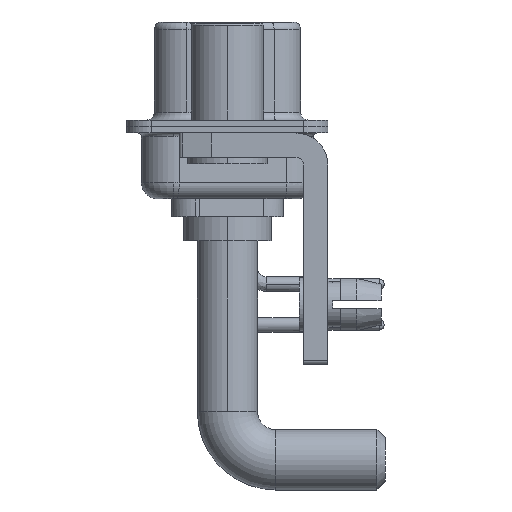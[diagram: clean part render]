
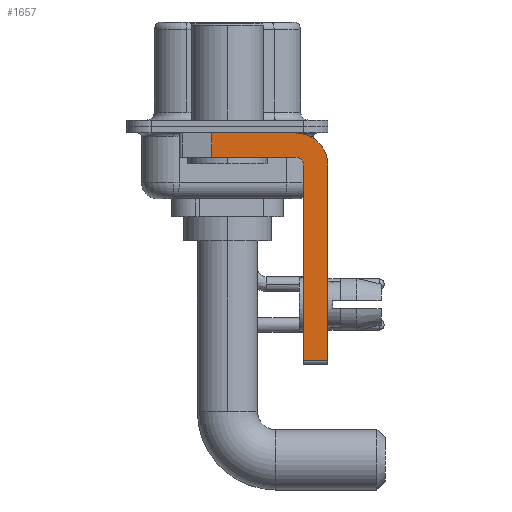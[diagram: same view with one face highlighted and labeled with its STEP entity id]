
A CAD part, left-side view. The second image highlights one B-rep face of the part: STEP entity #1657.
In plain terms, the highlighted planar face has unit normal (-1, 0, 0).
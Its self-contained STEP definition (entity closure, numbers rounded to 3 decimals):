
#322 = CARTESIAN_POINT ( 'NONE',  ( -2.9, -4.25, -1.9 ) ) ;
#999 = DIRECTION ( 'NONE',  ( 1., 0., 0. ) ) ;
#1108 = ORIENTED_EDGE ( 'NONE', *, *, #8049, .F. ) ;
#1657 = ADVANCED_FACE ( 'NONE', ( #18052 ), #25677, .F. ) ;
#1664 = CARTESIAN_POINT ( 'NONE',  ( -2.9, 0.978, -0.4 ) ) ;
#1812 = ORIENTED_EDGE ( 'NONE', *, *, #9223, .T. ) ;
#2180 = DIRECTION ( 'NONE',  ( 0., 0., -1. ) ) ;
#2213 = DIRECTION ( 'NONE',  ( 0., -1., 0. ) ) ;
#2520 = VERTEX_POINT ( 'NONE', #1664 ) ;
#2929 = CARTESIAN_POINT ( 'NONE',  ( -2.9, -4.25, -14.55 ) ) ;
#3032 = DIRECTION ( 'NONE',  ( 1., 0., 0. ) ) ;
#3142 = EDGE_LOOP ( 'NONE', ( #15228, #1812, #1108, #4092, #4650, #19514, #12246, #8804 ) ) ;
#3302 = CARTESIAN_POINT ( 'NONE',  ( -2.9, 0.978, -1.9 ) ) ;
#3963 = AXIS2_PLACEMENT_3D ( 'NONE', #21789, #3032, #10055 ) ;
#4092 = ORIENTED_EDGE ( 'NONE', *, *, #20405, .F. ) ;
#4118 = CARTESIAN_POINT ( 'NONE',  ( -2.9, -6.25, -14.55 ) ) ;
#4282 = CIRCLE ( 'NONE', #21753, 0.5 ) ;
#4650 = ORIENTED_EDGE ( 'NONE', *, *, #5585, .F. ) ;
#5585 = EDGE_CURVE ( 'NONE', #5754, #8852, #11050, .T. ) ;
#5587 = DIRECTION ( 'NONE',  ( 0., -1., 0. ) ) ;
#5754 = VERTEX_POINT ( 'NONE', #18016 ) ;
#6359 = DIRECTION ( 'NONE',  ( 0., 0., 1. ) ) ;
#8049 = EDGE_CURVE ( 'NONE', #29425, #20617, #15728, .T. ) ;
#8168 = DIRECTION ( 'NONE',  ( 0., 0., 1. ) ) ;
#8679 = CARTESIAN_POINT ( 'NONE',  ( -2.9, 0.978, -1.9 ) ) ;
#8804 = ORIENTED_EDGE ( 'NONE', *, *, #22685, .F. ) ;
#8818 = VECTOR ( 'NONE', #2213, 1000. ) ;
#8852 = VERTEX_POINT ( 'NONE', #23733 ) ;
#9223 = EDGE_CURVE ( 'NONE', #2520, #20617, #30101, .T. ) ;
#9384 = LINE ( 'NONE', #30484, #12333 ) ;
#9428 = AXIS2_PLACEMENT_3D ( 'NONE', #28188, #999, #27294 ) ;
#9888 = EDGE_CURVE ( 'NONE', #2520, #24561, #30674, .T. ) ;
#10055 = DIRECTION ( 'NONE',  ( 0., 0., -1. ) ) ;
#10423 = CARTESIAN_POINT ( 'NONE',  ( -2.9, -6.25, -2.4 ) ) ;
#11050 = LINE ( 'NONE', #20728, #16142 ) ;
#12246 = ORIENTED_EDGE ( 'NONE', *, *, #12914, .F. ) ;
#12333 = VECTOR ( 'NONE', #2180, 1000. ) ;
#12376 = CARTESIAN_POINT ( 'NONE',  ( -2.9, 3., -0.4 ) ) ;
#12457 = LINE ( 'NONE', #2929, #15855 ) ;
#12914 = EDGE_CURVE ( 'NONE', #25608, #18728, #9384, .T. ) ;
#13001 = CARTESIAN_POINT ( 'NONE',  ( -2.9, -4.25, -2.4 ) ) ;
#13775 = EDGE_CURVE ( 'NONE', #5754, #18728, #12457, .T. ) ;
#15228 = ORIENTED_EDGE ( 'NONE', *, *, #9888, .F. ) ;
#15265 = CARTESIAN_POINT ( 'NONE',  ( -2.9, -4.25, -1.9 ) ) ;
#15728 = LINE ( 'NONE', #15265, #21947 ) ;
#15855 = VECTOR ( 'NONE', #5587, 1000. ) ;
#16142 = VECTOR ( 'NONE', #6359, 1000. ) ;
#18016 = CARTESIAN_POINT ( 'NONE',  ( -2.9, -4.75, -14.55 ) ) ;
#18052 = FACE_OUTER_BOUND ( 'NONE', #3142, .T. ) ;
#18158 = CARTESIAN_POINT ( 'NONE',  ( -2.9, -4.25, -0.4 ) ) ;
#18465 = CIRCLE ( 'NONE', #3963, 2. ) ;
#18728 = VERTEX_POINT ( 'NONE', #4118 ) ;
#19514 = ORIENTED_EDGE ( 'NONE', *, *, #13775, .T. ) ;
#19955 = DIRECTION ( 'NONE',  ( 0., 0., -1. ) ) ;
#20114 = DIRECTION ( 'NONE',  ( 0., 1., 0. ) ) ;
#20405 = EDGE_CURVE ( 'NONE', #8852, #29425, #4282, .T. ) ;
#20617 = VERTEX_POINT ( 'NONE', #3302 ) ;
#20728 = CARTESIAN_POINT ( 'NONE',  ( -2.9, -4.75, -14.8 ) ) ;
#21753 = AXIS2_PLACEMENT_3D ( 'NONE', #13001, #23011, #8168 ) ;
#21789 = CARTESIAN_POINT ( 'NONE',  ( -2.9, -4.25, -2.4 ) ) ;
#21947 = VECTOR ( 'NONE', #20114, 1000. ) ;
#22685 = EDGE_CURVE ( 'NONE', #24561, #25608, #18465, .T. ) ;
#23011 = DIRECTION ( 'NONE',  ( -1., 0., 0. ) ) ;
#23733 = CARTESIAN_POINT ( 'NONE',  ( -2.9, -4.75, -2.4 ) ) ;
#24561 = VERTEX_POINT ( 'NONE', #18158 ) ;
#25608 = VERTEX_POINT ( 'NONE', #10423 ) ;
#25677 = PLANE ( 'NONE',  #9428 ) ;
#27294 = DIRECTION ( 'NONE',  ( 0., 0., -1. ) ) ;
#28188 = CARTESIAN_POINT ( 'NONE',  ( -2.9, -4.25, -2.4 ) ) ;
#28326 = VECTOR ( 'NONE', #19955, 1000. ) ;
#29425 = VERTEX_POINT ( 'NONE', #322 ) ;
#30101 = LINE ( 'NONE', #8679, #28326 ) ;
#30484 = CARTESIAN_POINT ( 'NONE',  ( -2.9, -6.25, -2.4 ) ) ;
#30674 = LINE ( 'NONE', #12376, #8818 ) ;
